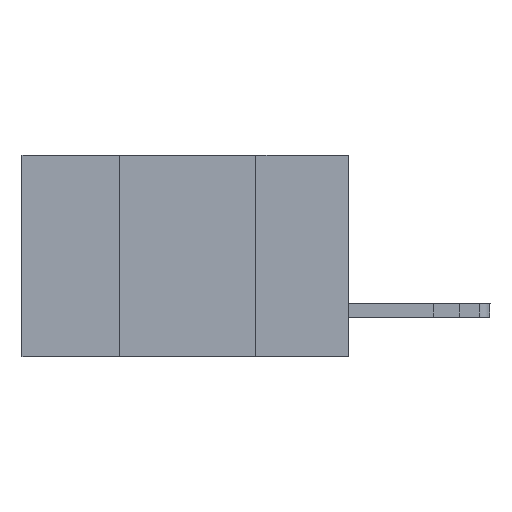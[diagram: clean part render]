
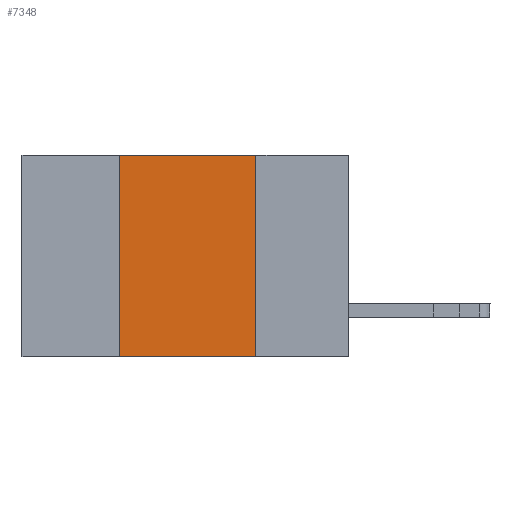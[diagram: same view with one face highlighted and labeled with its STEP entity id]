
A CAD part, left-side view. The second image highlights one B-rep face of the part: STEP entity #7348.
In plain terms, the highlighted planar face has unit normal (-1, 0, 0).
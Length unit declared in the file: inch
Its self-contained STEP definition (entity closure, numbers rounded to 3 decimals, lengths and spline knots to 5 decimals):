
#116 = CARTESIAN_POINT ( 'NONE',  ( 0., 0.42, -0.37 ) ) ;
#567 = VERTEX_POINT ( 'NONE', #6269 ) ;
#1378 = VECTOR ( 'NONE', #2664, 39.37008 ) ;
#2648 = LINE ( 'NONE', #14191, #3323 ) ;
#2664 = DIRECTION ( 'NONE',  ( 0., 0., 1. ) ) ;
#2672 = PLANE ( 'NONE',  #6340 ) ;
#2743 = CARTESIAN_POINT ( 'NONE',  ( 0., 0.6, 0. ) ) ;
#3251 = CARTESIAN_POINT ( 'NONE',  ( 0., 0.17, 0. ) ) ;
#3323 = VECTOR ( 'NONE', #16881, 39.37008 ) ;
#3563 = EDGE_LOOP ( 'NONE', ( #14342, #5327, #14149, #7608 ) ) ;
#4915 = VECTOR ( 'NONE', #5106, 39.37008 ) ;
#5106 = DIRECTION ( 'NONE',  ( 0., 0., -1. ) ) ;
#5327 = ORIENTED_EDGE ( 'NONE', *, *, #9575, .F. ) ;
#5926 = VECTOR ( 'NONE', #16798, 39.37008 ) ;
#6229 = LINE ( 'NONE', #10959, #4915 ) ;
#6269 = CARTESIAN_POINT ( 'NONE',  ( 0., 0.17, -0.37 ) ) ;
#6340 = AXIS2_PLACEMENT_3D ( 'NONE', #2743, #15386, #12653 ) ;
#7348 = ADVANCED_FACE ( 'NONE', ( #10260 ), #2672, .F. ) ;
#7608 = ORIENTED_EDGE ( 'NONE', *, *, #16093, .T. ) ;
#8224 = VERTEX_POINT ( 'NONE', #116 ) ;
#9539 = LINE ( 'NONE', #11060, #1378 ) ;
#9575 = EDGE_CURVE ( 'NONE', #13457, #16495, #2648, .T. ) ;
#10260 = FACE_OUTER_BOUND ( 'NONE', #3563, .T. ) ;
#10959 = CARTESIAN_POINT ( 'NONE',  ( 0., 0.17, 0. ) ) ;
#11060 = CARTESIAN_POINT ( 'NONE',  ( 0., 0.42, 0. ) ) ;
#12424 = CARTESIAN_POINT ( 'NONE',  ( 0., 0.6, -0.37 ) ) ;
#12653 = DIRECTION ( 'NONE',  ( 0., 0., -1. ) ) ;
#13093 = EDGE_CURVE ( 'NONE', #8224, #13457, #9539, .T. ) ;
#13314 = EDGE_CURVE ( 'NONE', #16495, #567, #6229, .T. ) ;
#13457 = VERTEX_POINT ( 'NONE', #15240 ) ;
#14149 = ORIENTED_EDGE ( 'NONE', *, *, #13093, .F. ) ;
#14191 = CARTESIAN_POINT ( 'NONE',  ( 0., 0.6, 0. ) ) ;
#14342 = ORIENTED_EDGE ( 'NONE', *, *, #13314, .F. ) ;
#15240 = CARTESIAN_POINT ( 'NONE',  ( 0., 0.42, 0. ) ) ;
#15386 = DIRECTION ( 'NONE',  ( 1., 0., 0. ) ) ;
#16093 = EDGE_CURVE ( 'NONE', #8224, #567, #17466, .T. ) ;
#16495 = VERTEX_POINT ( 'NONE', #3251 ) ;
#16798 = DIRECTION ( 'NONE',  ( 0., -1., 0. ) ) ;
#16881 = DIRECTION ( 'NONE',  ( 0., -1., 0. ) ) ;
#17466 = LINE ( 'NONE', #12424, #5926 ) ;
